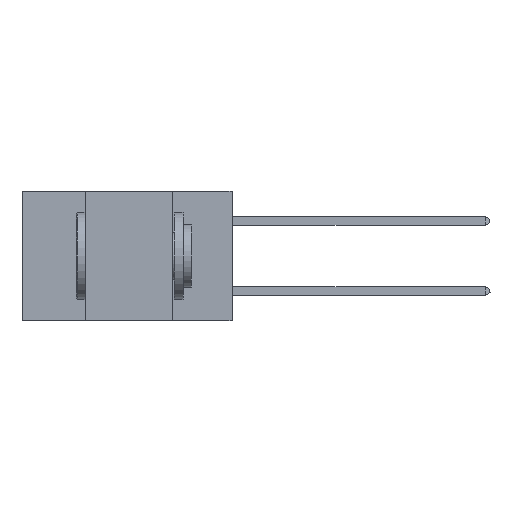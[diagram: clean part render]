
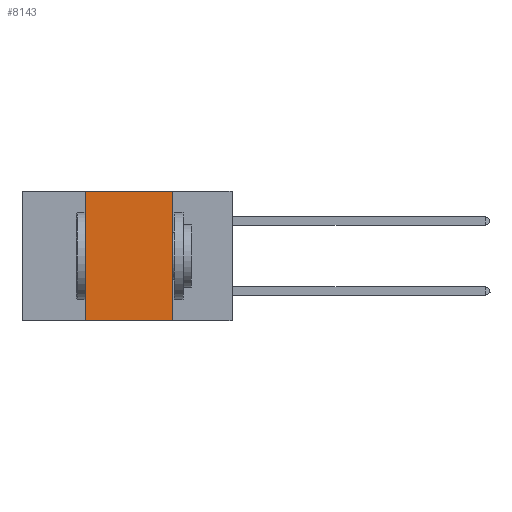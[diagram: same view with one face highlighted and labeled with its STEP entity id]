
A CAD part, left-side view. The second image highlights one B-rep face of the part: STEP entity #8143.
In plain terms, the highlighted planar face has unit normal (-1, 0, 0).
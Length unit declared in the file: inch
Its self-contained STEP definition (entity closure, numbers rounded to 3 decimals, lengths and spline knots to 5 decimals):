
#93 = CARTESIAN_POINT ( 'NONE',  ( 0., 0.17, 0. ) ) ;
#1847 = AXIS2_PLACEMENT_3D ( 'NONE', #4266, #32057, #4466 ) ;
#2350 = EDGE_CURVE ( 'NONE', #4159, #11494, #25420, .T. ) ;
#3233 = EDGE_CURVE ( 'NONE', #5227, #11494, #26099, .T. ) ;
#4159 = VERTEX_POINT ( 'NONE', #8805 ) ;
#4266 = CARTESIAN_POINT ( 'NONE',  ( 0., 0.6, 0. ) ) ;
#4466 = DIRECTION ( 'NONE',  ( 0., 0., -1. ) ) ;
#4843 = VECTOR ( 'NONE', #9618, 39.37008 ) ;
#5227 = VERTEX_POINT ( 'NONE', #10650 ) ;
#6258 = VECTOR ( 'NONE', #9354, 39.37008 ) ;
#6721 = EDGE_CURVE ( 'NONE', #5227, #21705, #15669, .T. ) ;
#8010 = LINE ( 'NONE', #31774, #27080 ) ;
#8143 = ADVANCED_FACE ( 'NONE', ( #12148 ), #21489, .F. ) ;
#8805 = CARTESIAN_POINT ( 'NONE',  ( 0., 0.17, 0. ) ) ;
#9354 = DIRECTION ( 'NONE',  ( 0., -1., 0. ) ) ;
#9618 = DIRECTION ( 'NONE',  ( 0., 0., 1. ) ) ;
#9864 = DIRECTION ( 'NONE',  ( 0., 0., -1. ) ) ;
#10650 = CARTESIAN_POINT ( 'NONE',  ( 0., 0.42, -0.37 ) ) ;
#11010 = VECTOR ( 'NONE', #9864, 39.37008 ) ;
#11494 = VERTEX_POINT ( 'NONE', #11495 ) ;
#11495 = CARTESIAN_POINT ( 'NONE',  ( 0., 0.17, -0.37 ) ) ;
#11645 = CARTESIAN_POINT ( 'NONE',  ( 0., 0.6, -0.37 ) ) ;
#12148 = FACE_OUTER_BOUND ( 'NONE', #27423, .T. ) ;
#15669 = LINE ( 'NONE', #22434, #4843 ) ;
#20352 = EDGE_CURVE ( 'NONE', #21705, #4159, #8010, .T. ) ;
#21489 = PLANE ( 'NONE',  #1847 ) ;
#21705 = VERTEX_POINT ( 'NONE', #24439 ) ;
#22434 = CARTESIAN_POINT ( 'NONE',  ( 0., 0.42, 0. ) ) ;
#22848 = ORIENTED_EDGE ( 'NONE', *, *, #20352, .F. ) ;
#24439 = CARTESIAN_POINT ( 'NONE',  ( 0., 0.42, 0. ) ) ;
#25420 = LINE ( 'NONE', #93, #11010 ) ;
#26099 = LINE ( 'NONE', #11645, #6258 ) ;
#27080 = VECTOR ( 'NONE', #32007, 39.37008 ) ;
#27108 = ORIENTED_EDGE ( 'NONE', *, *, #6721, .F. ) ;
#27423 = EDGE_LOOP ( 'NONE', ( #29237, #22848, #27108, #28501 ) ) ;
#28501 = ORIENTED_EDGE ( 'NONE', *, *, #3233, .T. ) ;
#29237 = ORIENTED_EDGE ( 'NONE', *, *, #2350, .F. ) ;
#31774 = CARTESIAN_POINT ( 'NONE',  ( 0., 0.6, 0. ) ) ;
#32007 = DIRECTION ( 'NONE',  ( 0., -1., 0. ) ) ;
#32057 = DIRECTION ( 'NONE',  ( 1., 0., 0. ) ) ;
